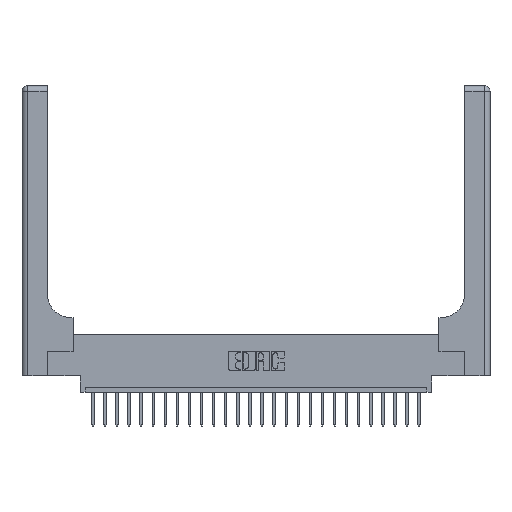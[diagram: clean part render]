
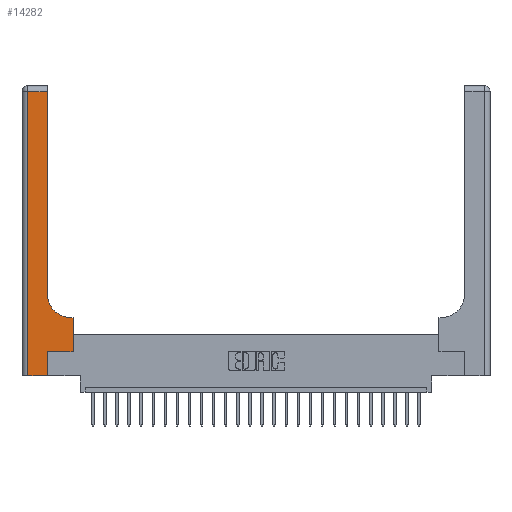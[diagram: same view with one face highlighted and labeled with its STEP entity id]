
A CAD part, top view. The second image highlights one B-rep face of the part: STEP entity #14282.
In plain terms, the highlighted planar face has unit normal (0, 0, 1).
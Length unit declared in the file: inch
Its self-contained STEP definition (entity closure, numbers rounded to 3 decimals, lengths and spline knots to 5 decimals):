
#475 = CARTESIAN_POINT ( 'NONE',  ( 0., 0., 0.37 ) ) ;
#840 = DIRECTION ( 'NONE',  ( 0., 1., 0. ) ) ;
#861 = LINE ( 'NONE', #5403, #12437 ) ;
#915 = CARTESIAN_POINT ( 'NONE',  ( 0.06, 0., 0.37 ) ) ;
#1160 = CARTESIAN_POINT ( 'NONE',  ( 0.528, 0.25, 0.37 ) ) ;
#1410 = VECTOR ( 'NONE', #840, 39.37008 ) ;
#1775 = CARTESIAN_POINT ( 'NONE',  ( 0.528, 0.6, 0.37 ) ) ;
#2544 = CARTESIAN_POINT ( 'NONE',  ( 0.51, 0.6, 0.37 ) ) ;
#3220 = EDGE_CURVE ( 'NONE', #14542, #3548, #861, .T. ) ;
#3548 = VERTEX_POINT ( 'NONE', #14081 ) ;
#3914 = EDGE_CURVE ( 'NONE', #21550, #20421, #21589, .T. ) ;
#4989 = VECTOR ( 'NONE', #18509, 39.37008 ) ;
#5012 = VECTOR ( 'NONE', #14088, 39.37008 ) ;
#5149 = DIRECTION ( 'NONE',  ( 0., 1., 0. ) ) ;
#5186 = ORIENTED_EDGE ( 'NONE', *, *, #19999, .T. ) ;
#5403 = CARTESIAN_POINT ( 'NONE',  ( 0.26, 3., 0.37 ) ) ;
#5642 = VECTOR ( 'NONE', #15401, 39.37008 ) ;
#5851 = CARTESIAN_POINT ( 'NONE',  ( 0.26, 0.6, 0.37 ) ) ;
#6258 = LINE ( 'NONE', #5851, #5642 ) ;
#6497 = LINE ( 'NONE', #16127, #1410 ) ;
#6896 = CARTESIAN_POINT ( 'NONE',  ( 0., 2.94, 0.37 ) ) ;
#6988 = LINE ( 'NONE', #1160, #20861 ) ;
#7193 = CARTESIAN_POINT ( 'NONE',  ( 0.51, 0.85, 0.37 ) ) ;
#7284 = EDGE_CURVE ( 'NONE', #11979, #20307, #19326, .T. ) ;
#7348 = ORIENTED_EDGE ( 'NONE', *, *, #22069, .T. ) ;
#9326 = DIRECTION ( 'NONE',  ( 0., 0., -1. ) ) ;
#10062 = LINE ( 'NONE', #23297, #5012 ) ;
#10596 = VERTEX_POINT ( 'NONE', #1775 ) ;
#10943 = VECTOR ( 'NONE', #12652, 39.37008 ) ;
#11419 = ORIENTED_EDGE ( 'NONE', *, *, #21531, .T. ) ;
#11534 = CARTESIAN_POINT ( 'NONE',  ( 0.528, 0.25, 0.37 ) ) ;
#11542 = LINE ( 'NONE', #6896, #10943 ) ;
#11979 = VERTEX_POINT ( 'NONE', #915 ) ;
#12184 = DIRECTION ( 'NONE',  ( -1., 0., 0. ) ) ;
#12437 = VECTOR ( 'NONE', #13573, 39.37008 ) ;
#12652 = DIRECTION ( 'NONE',  ( -1., 0., 0. ) ) ;
#13573 = DIRECTION ( 'NONE',  ( 0., 1., 0. ) ) ;
#13696 = FACE_OUTER_BOUND ( 'NONE', #17878, .T. ) ;
#13867 = AXIS2_PLACEMENT_3D ( 'NONE', #21548, #19726, #12184 ) ;
#14081 = CARTESIAN_POINT ( 'NONE',  ( 0.26, 2.94, 0.37 ) ) ;
#14088 = DIRECTION ( 'NONE',  ( 0., -1., 0. ) ) ;
#14282 = ADVANCED_FACE ( 'NONE', ( #13696 ), #23552, .F. ) ;
#14404 = VERTEX_POINT ( 'NONE', #2544 ) ;
#14542 = VERTEX_POINT ( 'NONE', #18470 ) ;
#15107 = EDGE_CURVE ( 'NONE', #14404, #14542, #18428, .T. ) ;
#15401 = DIRECTION ( 'NONE',  ( -1., 0., 0. ) ) ;
#16127 = CARTESIAN_POINT ( 'NONE',  ( 0.265, 0., 0.37 ) ) ;
#16584 = EDGE_CURVE ( 'NONE', #3548, #17967, #11542, .T. ) ;
#16895 = DIRECTION ( 'NONE',  ( 1., 0., 0. ) ) ;
#16907 = EDGE_CURVE ( 'NONE', #20307, #21550, #6497, .T. ) ;
#17850 = CARTESIAN_POINT ( 'NONE',  ( 0.265, 0.25, 0.37 ) ) ;
#17878 = EDGE_LOOP ( 'NONE', ( #17978, #22559, #7348, #19364, #20821, #20777, #5186, #11419, #18521 ) ) ;
#17967 = VERTEX_POINT ( 'NONE', #23949 ) ;
#17978 = ORIENTED_EDGE ( 'NONE', *, *, #3220, .T. ) ;
#18339 = AXIS2_PLACEMENT_3D ( 'NONE', #7193, #9326, #16895 ) ;
#18428 = CIRCLE ( 'NONE', #18339, 0.25 ) ;
#18470 = CARTESIAN_POINT ( 'NONE',  ( 0.26, 0.85, 0.37 ) ) ;
#18509 = DIRECTION ( 'NONE',  ( 1., 0., 0. ) ) ;
#18521 = ORIENTED_EDGE ( 'NONE', *, *, #15107, .T. ) ;
#19326 = LINE ( 'NONE', #475, #22896 ) ;
#19364 = ORIENTED_EDGE ( 'NONE', *, *, #7284, .T. ) ;
#19438 = CARTESIAN_POINT ( 'NONE',  ( 0.265, 0., 0.37 ) ) ;
#19726 = DIRECTION ( 'NONE',  ( 0., 0., -1. ) ) ;
#19999 = EDGE_CURVE ( 'NONE', #20421, #10596, #6988, .T. ) ;
#20307 = VERTEX_POINT ( 'NONE', #19438 ) ;
#20350 = CARTESIAN_POINT ( 'NONE',  ( 0.265, 0.25, 0.37 ) ) ;
#20421 = VERTEX_POINT ( 'NONE', #11534 ) ;
#20777 = ORIENTED_EDGE ( 'NONE', *, *, #3914, .T. ) ;
#20821 = ORIENTED_EDGE ( 'NONE', *, *, #16907, .T. ) ;
#20861 = VECTOR ( 'NONE', #5149, 39.37008 ) ;
#21050 = DIRECTION ( 'NONE',  ( 1., 0., 0. ) ) ;
#21531 = EDGE_CURVE ( 'NONE', #10596, #14404, #6258, .T. ) ;
#21548 = CARTESIAN_POINT ( 'NONE',  ( 0., 3., 0.37 ) ) ;
#21550 = VERTEX_POINT ( 'NONE', #17850 ) ;
#21589 = LINE ( 'NONE', #20350, #4989 ) ;
#22069 = EDGE_CURVE ( 'NONE', #17967, #11979, #10062, .T. ) ;
#22559 = ORIENTED_EDGE ( 'NONE', *, *, #16584, .T. ) ;
#22896 = VECTOR ( 'NONE', #21050, 39.37008 ) ;
#23297 = CARTESIAN_POINT ( 'NONE',  ( 0.06, 3., 0.37 ) ) ;
#23552 = PLANE ( 'NONE',  #13867 ) ;
#23949 = CARTESIAN_POINT ( 'NONE',  ( 0.06, 2.94, 0.37 ) ) ;
